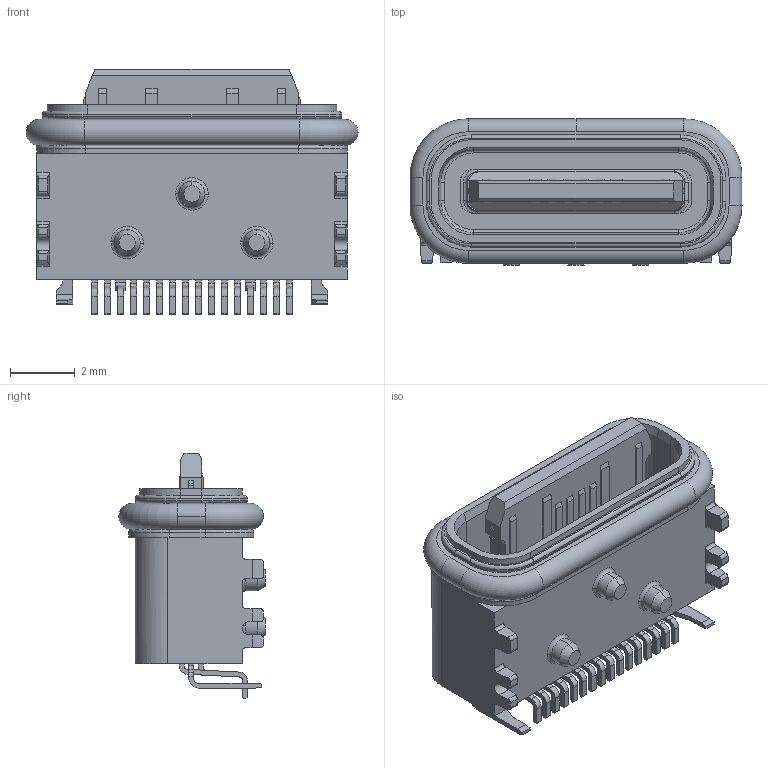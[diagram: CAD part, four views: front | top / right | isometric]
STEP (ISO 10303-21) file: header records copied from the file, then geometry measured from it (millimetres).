
FILE_DESCRIPTION (( 'STEP AP214' ), '1' );
FILE_NAME ('698B116W16A-661 - EDAC USB Connector.STEP', '2021-01-15T15:56:38', ( '' ), ( '' ), 'SwSTEP 2.0', 'SolidWorks 2020', '' );
FILE_SCHEMA (( 'AUTOMOTIVE_DESIGN' ));
Length unit declared in the file: millimetre
Products named in the file (1): 698B116W16A-661 - EDAC USB Connector
Bounding box: 10.24 x 4.51 x 7.58 mm (x, y, z)
Volume: 135.1 mm3; surface area: 430.1 mm2
Topology: 1 solids, 3 shells, 678 faces, 1868 edges, 1220 vertices
Faces by surface type: plane 420, cylinder 200, bspline 36, cone 18, torus 4
Entity records: 25240 total; most frequent: CARTESIAN_POINT 5778, ORIENTED_EDGE 3736, DIRECTION 3207, EDGE_CURVE 1868, LINE 1281, VECTOR 1281, VERTEX_POINT 1220, AXIS2_PLACEMENT_3D 963
